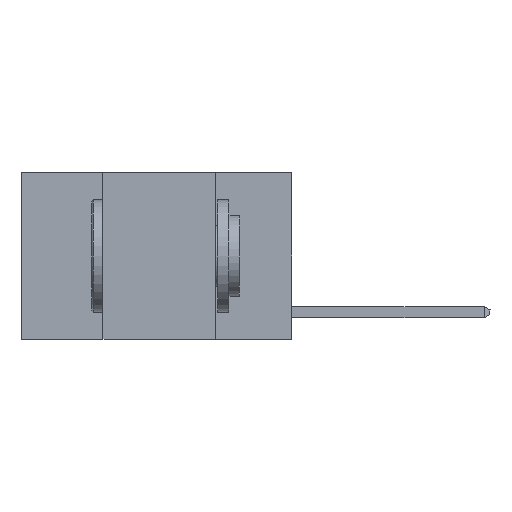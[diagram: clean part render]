
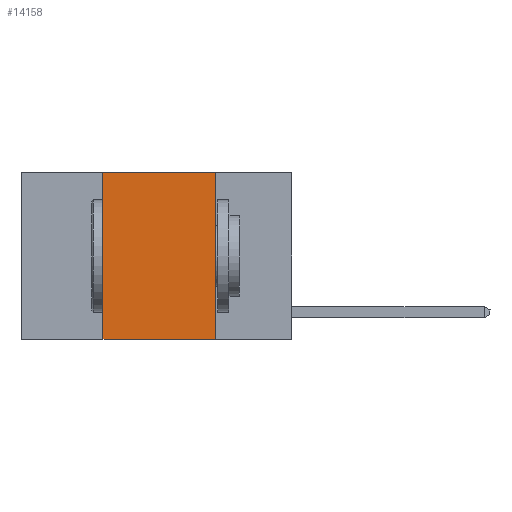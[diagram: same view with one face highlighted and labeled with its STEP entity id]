
A CAD part, left-side view. The second image highlights one B-rep face of the part: STEP entity #14158.
In plain terms, the highlighted planar face has unit normal (-1, 0, 0).
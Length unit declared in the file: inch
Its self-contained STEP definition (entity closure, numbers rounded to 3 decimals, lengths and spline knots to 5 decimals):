
#1121 = CARTESIAN_POINT ( 'NONE',  ( 0., 0.42, 0. ) ) ;
#1561 = VERTEX_POINT ( 'NONE', #20446 ) ;
#2071 = EDGE_CURVE ( 'NONE', #1561, #20006, #19873, .T. ) ;
#2421 = LINE ( 'NONE', #5825, #7036 ) ;
#2503 = VECTOR ( 'NONE', #3564, 39.37008 ) ;
#3564 = DIRECTION ( 'NONE',  ( 0., 0., 1. ) ) ;
#3658 = CARTESIAN_POINT ( 'NONE',  ( 0., 0.17, 0. ) ) ;
#3826 = EDGE_CURVE ( 'NONE', #23963, #16300, #20400, .T. ) ;
#4204 = CARTESIAN_POINT ( 'NONE',  ( 0., 0.6, -0.37 ) ) ;
#4270 = CARTESIAN_POINT ( 'NONE',  ( 0., 0.17, -0.37 ) ) ;
#4419 = PLANE ( 'NONE',  #25266 ) ;
#5334 = CARTESIAN_POINT ( 'NONE',  ( 0., 0.6, 0. ) ) ;
#5825 = CARTESIAN_POINT ( 'NONE',  ( 0., 0.17, 0. ) ) ;
#7036 = VECTOR ( 'NONE', #23475, 39.37008 ) ;
#7360 = DIRECTION ( 'NONE',  ( 0., -1., 0. ) ) ;
#8133 = DIRECTION ( 'NONE',  ( 0., -1., 0. ) ) ;
#8176 = ORIENTED_EDGE ( 'NONE', *, *, #11245, .F. ) ;
#8330 = CARTESIAN_POINT ( 'NONE',  ( 0., 0.6, 0. ) ) ;
#9293 = VECTOR ( 'NONE', #7360, 39.37008 ) ;
#9353 = CARTESIAN_POINT ( 'NONE',  ( 0., 0.42, 0. ) ) ;
#10291 = DIRECTION ( 'NONE',  ( 0., 0., -1. ) ) ;
#11245 = EDGE_CURVE ( 'NONE', #1561, #23963, #22771, .T. ) ;
#12153 = ORIENTED_EDGE ( 'NONE', *, *, #12565, .F. ) ;
#12565 = EDGE_CURVE ( 'NONE', #16300, #20006, #2421, .T. ) ;
#13378 = ORIENTED_EDGE ( 'NONE', *, *, #2071, .T. ) ;
#14158 = ADVANCED_FACE ( 'NONE', ( #21091 ), #4419, .F. ) ;
#15240 = VECTOR ( 'NONE', #8133, 39.37008 ) ;
#16300 = VERTEX_POINT ( 'NONE', #3658 ) ;
#18040 = ORIENTED_EDGE ( 'NONE', *, *, #3826, .F. ) ;
#19873 = LINE ( 'NONE', #4204, #15240 ) ;
#20006 = VERTEX_POINT ( 'NONE', #4270 ) ;
#20400 = LINE ( 'NONE', #5334, #9293 ) ;
#20446 = CARTESIAN_POINT ( 'NONE',  ( 0., 0.42, -0.37 ) ) ;
#21091 = FACE_OUTER_BOUND ( 'NONE', #21247, .T. ) ;
#21247 = EDGE_LOOP ( 'NONE', ( #12153, #18040, #8176, #13378 ) ) ;
#22069 = DIRECTION ( 'NONE',  ( 1., 0., 0. ) ) ;
#22771 = LINE ( 'NONE', #9353, #2503 ) ;
#23475 = DIRECTION ( 'NONE',  ( 0., 0., -1. ) ) ;
#23963 = VERTEX_POINT ( 'NONE', #1121 ) ;
#25266 = AXIS2_PLACEMENT_3D ( 'NONE', #8330, #22069, #10291 ) ;
